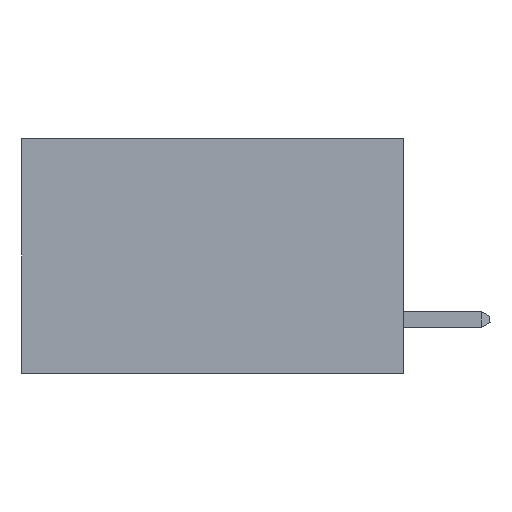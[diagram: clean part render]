
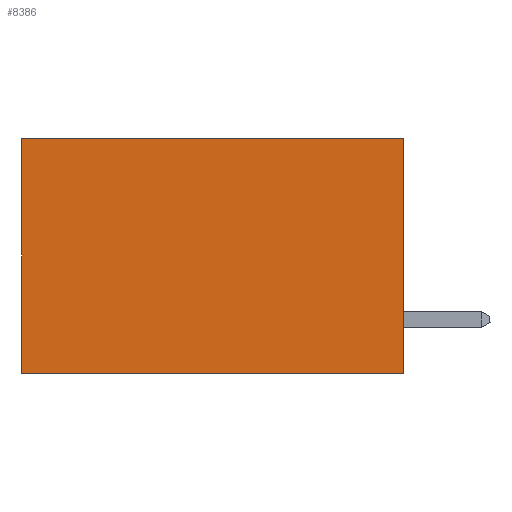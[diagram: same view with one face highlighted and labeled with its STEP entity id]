
A CAD part, left-side view. The second image highlights one B-rep face of the part: STEP entity #8386.
In plain terms, the highlighted planar face has unit normal (-1, 0, 0).
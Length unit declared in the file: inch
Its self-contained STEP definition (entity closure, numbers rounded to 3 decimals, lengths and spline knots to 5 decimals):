
#346 = EDGE_CURVE ( 'NONE', #9801, #23064, #17035, .T. ) ;
#1570 = CARTESIAN_POINT ( 'NONE',  ( 0.2875, 0., -0.37 ) ) ;
#2358 = VECTOR ( 'NONE', #14962, 39.37008 ) ;
#2780 = DIRECTION ( 'NONE',  ( 0., 0., -1. ) ) ;
#3350 = ORIENTED_EDGE ( 'NONE', *, *, #346, .F. ) ;
#5356 = AXIS2_PLACEMENT_3D ( 'NONE', #17395, #23084, #2780 ) ;
#5495 = CARTESIAN_POINT ( 'NONE',  ( 0.2875, 0., 0. ) ) ;
#5854 = LINE ( 'NONE', #18716, #2358 ) ;
#6586 = EDGE_CURVE ( 'NONE', #23064, #13240, #23245, .T. ) ;
#7039 = DIRECTION ( 'NONE',  ( 0., 1., 0. ) ) ;
#7207 = ORIENTED_EDGE ( 'NONE', *, *, #13633, .T. ) ;
#7520 = ORIENTED_EDGE ( 'NONE', *, *, #7990, .T. ) ;
#7990 = EDGE_CURVE ( 'NONE', #9241, #13240, #5854, .T. ) ;
#8386 = ADVANCED_FACE ( 'NONE', ( #12462 ), #18560, .F. ) ;
#8934 = VECTOR ( 'NONE', #20129, 39.37008 ) ;
#9241 = VERTEX_POINT ( 'NONE', #13596 ) ;
#9801 = VERTEX_POINT ( 'NONE', #19962 ) ;
#11640 = CARTESIAN_POINT ( 'NONE',  ( 0.2875, 0., 0. ) ) ;
#11673 = CARTESIAN_POINT ( 'NONE',  ( 0.2875, 0., -0.37 ) ) ;
#12462 = FACE_OUTER_BOUND ( 'NONE', #18220, .T. ) ;
#13240 = VERTEX_POINT ( 'NONE', #22521 ) ;
#13547 = LINE ( 'NONE', #11640, #14974 ) ;
#13596 = CARTESIAN_POINT ( 'NONE',  ( 0.2875, 0.6, 0. ) ) ;
#13633 = EDGE_CURVE ( 'NONE', #9801, #9241, #13547, .T. ) ;
#13984 = DIRECTION ( 'NONE',  ( 0., 1., 0. ) ) ;
#14962 = DIRECTION ( 'NONE',  ( 0., 0., -1. ) ) ;
#14974 = VECTOR ( 'NONE', #13984, 39.37008 ) ;
#17035 = LINE ( 'NONE', #5495, #8934 ) ;
#17395 = CARTESIAN_POINT ( 'NONE',  ( 0.2875, 0., 0. ) ) ;
#18220 = EDGE_LOOP ( 'NONE', ( #7520, #21031, #3350, #7207 ) ) ;
#18560 = PLANE ( 'NONE',  #5356 ) ;
#18716 = CARTESIAN_POINT ( 'NONE',  ( 0.2875, 0.6, 0. ) ) ;
#19962 = CARTESIAN_POINT ( 'NONE',  ( 0.2875, 0., 0. ) ) ;
#20129 = DIRECTION ( 'NONE',  ( 0., 0., -1. ) ) ;
#21031 = ORIENTED_EDGE ( 'NONE', *, *, #6586, .F. ) ;
#21243 = VECTOR ( 'NONE', #7039, 39.37008 ) ;
#22521 = CARTESIAN_POINT ( 'NONE',  ( 0.2875, 0.6, -0.37 ) ) ;
#23064 = VERTEX_POINT ( 'NONE', #11673 ) ;
#23084 = DIRECTION ( 'NONE',  ( 1., 0., 0. ) ) ;
#23245 = LINE ( 'NONE', #1570, #21243 ) ;
